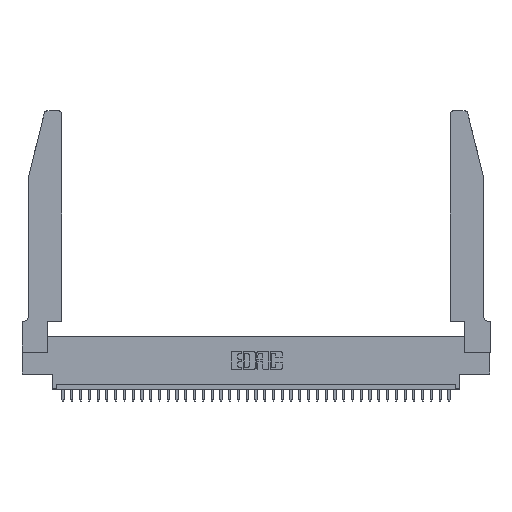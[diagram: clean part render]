
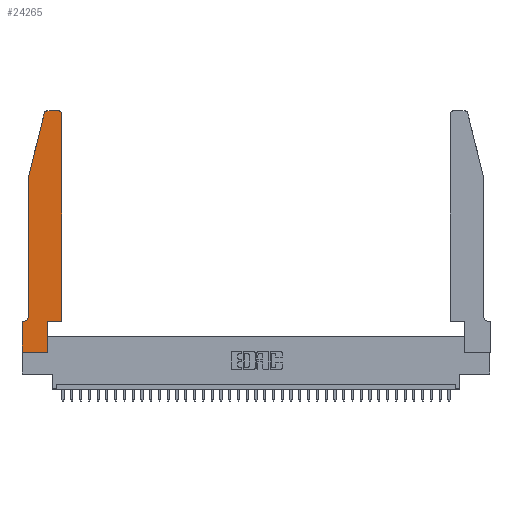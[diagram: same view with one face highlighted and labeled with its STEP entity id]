
A CAD part, top view. The second image highlights one B-rep face of the part: STEP entity #24265.
In plain terms, the highlighted planar face has unit normal (0, 0, 1).
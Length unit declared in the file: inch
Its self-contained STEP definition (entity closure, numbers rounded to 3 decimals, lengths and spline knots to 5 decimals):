
#1338 = ORIENTED_EDGE ( 'NONE', *, *, #5486, .T. ) ;
#1914 = CARTESIAN_POINT ( 'NONE',  ( 0.4505, 0.35, 0.37 ) ) ;
#1973 = DIRECTION ( 'NONE',  ( 0., -1., 0. ) ) ;
#2005 = DIRECTION ( 'NONE',  ( 1., 0., 0. ) ) ;
#2288 = DIRECTION ( 'NONE',  ( 1., 0., 0. ) ) ;
#2460 = CARTESIAN_POINT ( 'NONE',  ( 0.25487, 2.72718, 0.37 ) ) ;
#2955 = EDGE_CURVE ( 'NONE', #3206, #16048, #3518, .T. ) ;
#2967 = ORIENTED_EDGE ( 'NONE', *, *, #4161, .T. ) ;
#3206 = VERTEX_POINT ( 'NONE', #2460 ) ;
#3518 = LINE ( 'NONE', #5213, #10524 ) ;
#3723 = PLANE ( 'NONE',  #31641 ) ;
#4161 = EDGE_CURVE ( 'NONE', #20325, #5856, #33599, .T. ) ;
#4471 = CARTESIAN_POINT ( 'NONE',  ( 0.4205, 2.75, 0.37 ) ) ;
#5102 = ORIENTED_EDGE ( 'NONE', *, *, #2955, .T. ) ;
#5213 = CARTESIAN_POINT ( 'NONE',  ( 0.0755, 2., 0.37 ) ) ;
#5397 = CARTESIAN_POINT ( 'NONE',  ( 0.0755, 2., 0.37 ) ) ;
#5486 = EDGE_CURVE ( 'NONE', #5856, #31889, #7966, .T. ) ;
#5856 = VERTEX_POINT ( 'NONE', #26715 ) ;
#6005 = CIRCLE ( 'NONE', #35597, 0.03 ) ;
#6163 = VECTOR ( 'NONE', #37714, 39.37008 ) ;
#7297 = EDGE_CURVE ( 'NONE', #18955, #32369, #18428, .T. ) ;
#7966 = LINE ( 'NONE', #9856, #26095 ) ;
#8007 = VERTEX_POINT ( 'NONE', #9656 ) ;
#8023 = VERTEX_POINT ( 'NONE', #24473 ) ;
#9363 = LINE ( 'NONE', #35107, #6163 ) ;
#9656 = CARTESIAN_POINT ( 'NONE',  ( 0.0755, 0.42, 0.37 ) ) ;
#9663 = CARTESIAN_POINT ( 'NONE',  ( 0.2605, 2.75, 0.37 ) ) ;
#9856 = CARTESIAN_POINT ( 'NONE',  ( 0., 0., 0.37 ) ) ;
#10277 = DIRECTION ( 'NONE',  ( 1., 0., 0. ) ) ;
#10366 = CIRCLE ( 'NONE', #13462, 0.03 ) ;
#10524 = VECTOR ( 'NONE', #31926, 39.37008 ) ;
#10826 = CARTESIAN_POINT ( 'NONE',  ( 0.284, 2.75, 0.37 ) ) ;
#11053 = DIRECTION ( 'NONE',  ( -1., 0., 0. ) ) ;
#12192 = AXIS2_PLACEMENT_3D ( 'NONE', #35133, #17145, #11053 ) ;
#12213 = EDGE_CURVE ( 'NONE', #8023, #25997, #26111, .T. ) ;
#12991 = CARTESIAN_POINT ( 'NONE',  ( 0.4505, 0.35, 0.37 ) ) ;
#13462 = AXIS2_PLACEMENT_3D ( 'NONE', #20063, #14335, #2288 ) ;
#13695 = CARTESIAN_POINT ( 'NONE',  ( 0.284, 2.72, 0.37 ) ) ;
#13850 = CARTESIAN_POINT ( 'NONE',  ( 0.0055, 0.35, 0.37 ) ) ;
#14335 = DIRECTION ( 'NONE',  ( 0., 0., 1. ) ) ;
#15492 = VECTOR ( 'NONE', #2005, 39.37008 ) ;
#15790 = DIRECTION ( 'NONE',  ( -1., 0., 0. ) ) ;
#15803 = DIRECTION ( 'NONE',  ( -1., 0., 0. ) ) ;
#16048 = VERTEX_POINT ( 'NONE', #5397 ) ;
#16105 = EDGE_CURVE ( 'NONE', #29152, #18955, #10366, .T. ) ;
#16671 = DIRECTION ( 'NONE',  ( 0., 0., 1. ) ) ;
#17145 = DIRECTION ( 'NONE',  ( 0., 0., -1. ) ) ;
#17585 = VERTEX_POINT ( 'NONE', #12991 ) ;
#17595 = EDGE_CURVE ( 'NONE', #16048, #8007, #33883, .T. ) ;
#18131 = VECTOR ( 'NONE', #31816, 39.37008 ) ;
#18428 = LINE ( 'NONE', #9663, #33290 ) ;
#18955 = VERTEX_POINT ( 'NONE', #4471 ) ;
#19667 = CARTESIAN_POINT ( 'NONE',  ( 0.2865, 0.35, 0.37 ) ) ;
#19677 = ORIENTED_EDGE ( 'NONE', *, *, #7297, .T. ) ;
#19728 = EDGE_CURVE ( 'NONE', #32369, #3206, #6005, .T. ) ;
#19794 = DIRECTION ( 'NONE',  ( 1., 0., 0. ) ) ;
#19949 = CARTESIAN_POINT ( 'NONE',  ( 0.2865, 0.35, 0.37 ) ) ;
#20063 = CARTESIAN_POINT ( 'NONE',  ( 0.4205, 2.72, 0.37 ) ) ;
#20325 = VERTEX_POINT ( 'NONE', #13850 ) ;
#20451 = CIRCLE ( 'NONE', #12192, 0.07 ) ;
#21287 = ORIENTED_EDGE ( 'NONE', *, *, #17595, .T. ) ;
#21638 = CARTESIAN_POINT ( 'NONE',  ( 0.0755, 0.35, 0.37 ) ) ;
#22076 = DIRECTION ( 'NONE',  ( 0., -1., 0. ) ) ;
#22380 = CARTESIAN_POINT ( 'NONE',  ( 0., 0., 0.37 ) ) ;
#22611 = CARTESIAN_POINT ( 'NONE',  ( 0.0755, 2., 0.37 ) ) ;
#22971 = VECTOR ( 'NONE', #15803, 39.37008 ) ;
#23257 = EDGE_LOOP ( 'NONE', ( #19677, #34733, #5102, #21287, #24668, #2967, #1338, #38188, #24481, #35573, #24215, #25025 ) ) ;
#23294 = LINE ( 'NONE', #1914, #27936 ) ;
#24215 = ORIENTED_EDGE ( 'NONE', *, *, #35309, .T. ) ;
#24265 = ADVANCED_FACE ( 'NONE', ( #26678 ), #3723, .T. ) ;
#24473 = CARTESIAN_POINT ( 'NONE',  ( 0.2865, 0., 0.37 ) ) ;
#24481 = ORIENTED_EDGE ( 'NONE', *, *, #12213, .T. ) ;
#24668 = ORIENTED_EDGE ( 'NONE', *, *, #35930, .T. ) ;
#25025 = ORIENTED_EDGE ( 'NONE', *, *, #16105, .T. ) ;
#25159 = EDGE_CURVE ( 'NONE', #25997, #17585, #9363, .T. ) ;
#25997 = VERTEX_POINT ( 'NONE', #19949 ) ;
#26095 = VECTOR ( 'NONE', #22076, 39.37008 ) ;
#26111 = LINE ( 'NONE', #19667, #18131 ) ;
#26227 = LINE ( 'NONE', #22380, #15492 ) ;
#26678 = FACE_OUTER_BOUND ( 'NONE', #23257, .T. ) ;
#26715 = CARTESIAN_POINT ( 'NONE',  ( 0., 0.35, 0.37 ) ) ;
#27427 = EDGE_CURVE ( 'NONE', #31889, #8023, #26227, .T. ) ;
#27936 = VECTOR ( 'NONE', #34682, 39.37008 ) ;
#29152 = VERTEX_POINT ( 'NONE', #32997 ) ;
#31641 = AXIS2_PLACEMENT_3D ( 'NONE', #34907, #37875, #10277 ) ;
#31816 = DIRECTION ( 'NONE',  ( 0., 1., 0. ) ) ;
#31889 = VERTEX_POINT ( 'NONE', #34574 ) ;
#31926 = DIRECTION ( 'NONE',  ( -0.239, -0.971, 0. ) ) ;
#32369 = VERTEX_POINT ( 'NONE', #10826 ) ;
#32997 = CARTESIAN_POINT ( 'NONE',  ( 0.4505, 2.72, 0.37 ) ) ;
#33290 = VECTOR ( 'NONE', #15790, 39.37008 ) ;
#33599 = LINE ( 'NONE', #21638, #22971 ) ;
#33883 = LINE ( 'NONE', #22611, #36685 ) ;
#34574 = CARTESIAN_POINT ( 'NONE',  ( 0., 0., 0.37 ) ) ;
#34682 = DIRECTION ( 'NONE',  ( 0., 1., 0. ) ) ;
#34733 = ORIENTED_EDGE ( 'NONE', *, *, #19728, .T. ) ;
#34907 = CARTESIAN_POINT ( 'NONE',  ( 0., 0.35, 0.37 ) ) ;
#35107 = CARTESIAN_POINT ( 'NONE',  ( 0.4505, 0.35, 0.37 ) ) ;
#35133 = CARTESIAN_POINT ( 'NONE',  ( 0.0055, 0.42, 0.37 ) ) ;
#35309 = EDGE_CURVE ( 'NONE', #17585, #29152, #23294, .T. ) ;
#35573 = ORIENTED_EDGE ( 'NONE', *, *, #25159, .T. ) ;
#35597 = AXIS2_PLACEMENT_3D ( 'NONE', #13695, #16671, #19794 ) ;
#35930 = EDGE_CURVE ( 'NONE', #8007, #20325, #20451, .T. ) ;
#36685 = VECTOR ( 'NONE', #1973, 39.37008 ) ;
#37714 = DIRECTION ( 'NONE',  ( 1., 0., 0. ) ) ;
#37875 = DIRECTION ( 'NONE',  ( 0., 0., 1. ) ) ;
#38188 = ORIENTED_EDGE ( 'NONE', *, *, #27427, .T. ) ;
